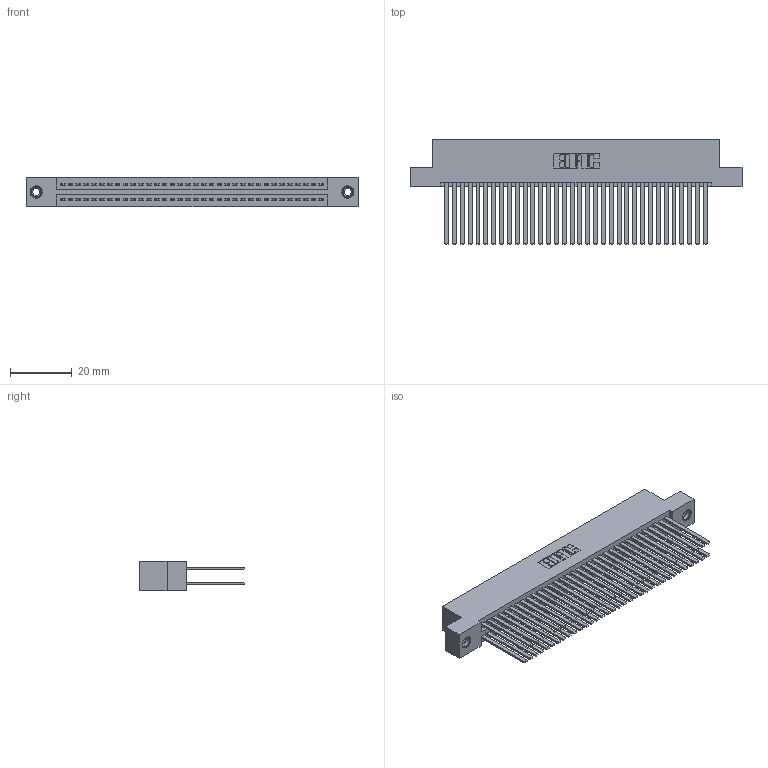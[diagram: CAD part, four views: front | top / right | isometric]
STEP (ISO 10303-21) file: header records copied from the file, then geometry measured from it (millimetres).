
FILE_DESCRIPTION (( 'STEP AP203' ), '1' );
FILE_NAME ('345-068-544-208.STEP', '2018-09-30T13:42:56', ( '' ), ( '' ), 'SwSTEP 2.0', 'SolidWorks 2016', '' );
FILE_SCHEMA (( 'CONFIG_CONTROL_DESIGN' ));
Length unit declared in the file: inch
Products named in the file (4): 345-250-001_345-250-003-102; 345-068-544-208; 345 Part_Flush Mounting Lugs - 0.156 Dia-TI; 345-292-001_345-293-144
Assembly tree (71 placements, depth 2):
  345-068-544-208
    345 Part_Flush Mounting Lugs - 0.156 Dia-TI
    345-292-001_345-293-144  x68
    345-250-001_345-250-003-102  x2
Bounding box: 107.57 x 33.96 x 9.4 mm (x, y, z)
Volume: 11321.8 mm3; surface area: 19387.9 mm2
Topology: 71 solids, 71 shells, 3178 faces, 9385 edges, 6158 vertices
Faces by surface type: plane 2084, cylinder 1078, cone 12, torus 4
Entity records: 28756 total; most frequent: CARTESIAN_POINT 4807, ORIENTED_EDGE 4734, DIRECTION 4273, EDGE_CURVE 2367, VECTOR 2083, LINE 2083, VERTEX_POINT 1572, AXIS2_PLACEMENT_3D 1095
